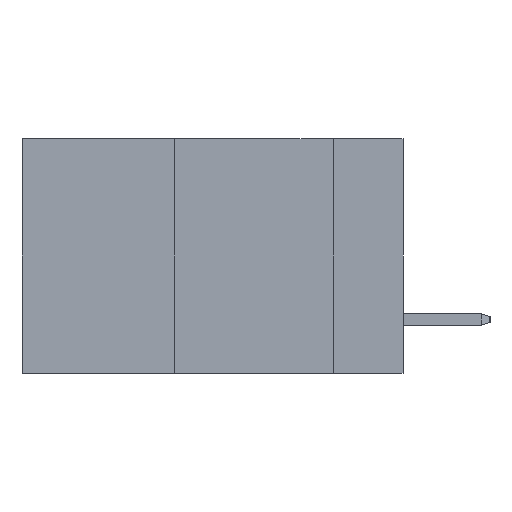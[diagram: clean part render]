
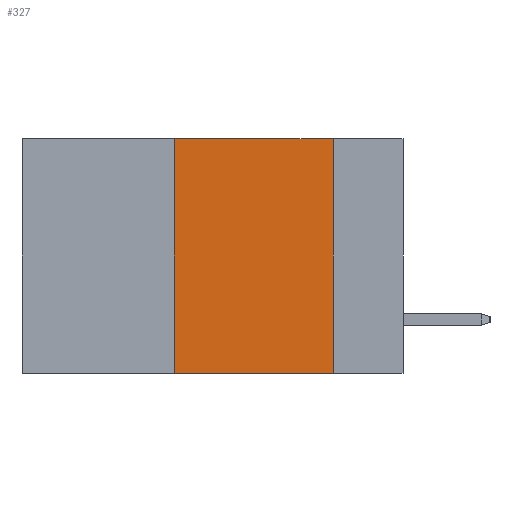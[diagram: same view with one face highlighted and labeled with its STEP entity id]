
A CAD part, left-side view. The second image highlights one B-rep face of the part: STEP entity #327.
In plain terms, the highlighted planar face has unit normal (-1, 0, 0).
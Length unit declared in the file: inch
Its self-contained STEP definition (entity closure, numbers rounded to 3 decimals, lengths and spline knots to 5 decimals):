
#327 = ADVANCED_FACE ( 'NONE', ( #30179 ), #2660, .F. ) ;
#704 = DIRECTION ( 'NONE',  ( 0., 0., -1. ) ) ;
#1004 = VERTEX_POINT ( 'NONE', #9354 ) ;
#1746 = VERTEX_POINT ( 'NONE', #28733 ) ;
#2660 = PLANE ( 'NONE',  #9294 ) ;
#2850 = CARTESIAN_POINT ( 'NONE',  ( 0., 0.11, -0.37 ) ) ;
#3293 = DIRECTION ( 'NONE',  ( 1., 0., 0. ) ) ;
#3469 = EDGE_CURVE ( 'NONE', #1746, #9182, #22042, .T. ) ;
#4515 = ORIENTED_EDGE ( 'NONE', *, *, #28905, .F. ) ;
#4919 = EDGE_CURVE ( 'NONE', #1004, #28766, #25444, .T. ) ;
#5300 = DIRECTION ( 'NONE',  ( 0., 0., -1. ) ) ;
#5647 = VECTOR ( 'NONE', #21190, 39.37008 ) ;
#5768 = CARTESIAN_POINT ( 'NONE',  ( 0., 0.11, 0. ) ) ;
#6809 = ORIENTED_EDGE ( 'NONE', *, *, #4919, .F. ) ;
#8014 = ORIENTED_EDGE ( 'NONE', *, *, #27647, .T. ) ;
#8944 = CARTESIAN_POINT ( 'NONE',  ( 0., 0.6, -0.37 ) ) ;
#9182 = VERTEX_POINT ( 'NONE', #15344 ) ;
#9294 = AXIS2_PLACEMENT_3D ( 'NONE', #17624, #3293, #704 ) ;
#9354 = CARTESIAN_POINT ( 'NONE',  ( 0., 0.11, 0. ) ) ;
#9499 = DIRECTION ( 'NONE',  ( 0., 0., 1. ) ) ;
#13286 = CARTESIAN_POINT ( 'NONE',  ( 0., 0.6, 0. ) ) ;
#13436 = VECTOR ( 'NONE', #30065, 39.37008 ) ;
#15344 = CARTESIAN_POINT ( 'NONE',  ( 0., 0.36, 0. ) ) ;
#16363 = EDGE_LOOP ( 'NONE', ( #6809, #4515, #18568, #8014 ) ) ;
#17624 = CARTESIAN_POINT ( 'NONE',  ( 0., 0.6, 0. ) ) ;
#18568 = ORIENTED_EDGE ( 'NONE', *, *, #3469, .F. ) ;
#19631 = CARTESIAN_POINT ( 'NONE',  ( 0., 0.36, 0. ) ) ;
#21190 = DIRECTION ( 'NONE',  ( 0., -1., 0. ) ) ;
#22042 = LINE ( 'NONE', #19631, #29497 ) ;
#23580 = VECTOR ( 'NONE', #5300, 39.37008 ) ;
#25444 = LINE ( 'NONE', #5768, #23580 ) ;
#25550 = LINE ( 'NONE', #13286, #13436 ) ;
#26175 = LINE ( 'NONE', #8944, #5647 ) ;
#27647 = EDGE_CURVE ( 'NONE', #1746, #28766, #26175, .T. ) ;
#28733 = CARTESIAN_POINT ( 'NONE',  ( 0., 0.36, -0.37 ) ) ;
#28766 = VERTEX_POINT ( 'NONE', #2850 ) ;
#28905 = EDGE_CURVE ( 'NONE', #9182, #1004, #25550, .T. ) ;
#29497 = VECTOR ( 'NONE', #9499, 39.37008 ) ;
#30065 = DIRECTION ( 'NONE',  ( 0., -1., 0. ) ) ;
#30179 = FACE_OUTER_BOUND ( 'NONE', #16363, .T. ) ;
